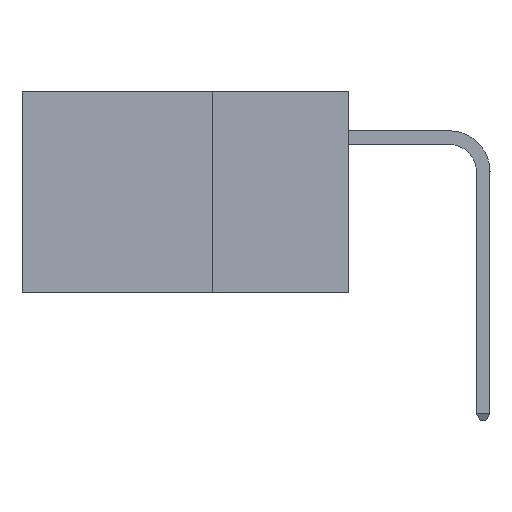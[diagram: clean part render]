
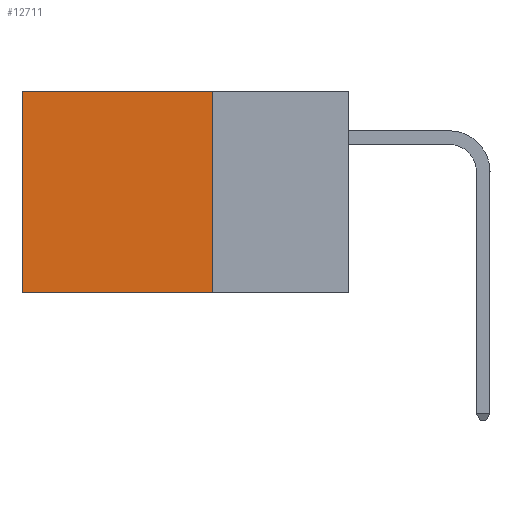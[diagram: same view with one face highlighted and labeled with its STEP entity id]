
A CAD part, left-side view. The second image highlights one B-rep face of the part: STEP entity #12711.
In plain terms, the highlighted planar face has unit normal (-1, 0, 0).
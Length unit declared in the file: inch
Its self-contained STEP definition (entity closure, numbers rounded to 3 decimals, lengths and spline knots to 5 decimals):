
#308 = EDGE_LOOP ( 'NONE', ( #20492, #718, #16041, #16776 ) ) ;
#398 = VERTEX_POINT ( 'NONE', #2685 ) ;
#718 = ORIENTED_EDGE ( 'NONE', *, *, #15885, .F. ) ;
#1490 = VECTOR ( 'NONE', #13937, 39.37008 ) ;
#2306 = CARTESIAN_POINT ( 'NONE',  ( 0.2875, 0.25, 0. ) ) ;
#2685 = CARTESIAN_POINT ( 'NONE',  ( 0.2875, 0.25, 0. ) ) ;
#4040 = DIRECTION ( 'NONE',  ( 0., 0., -1. ) ) ;
#4155 = EDGE_CURVE ( 'NONE', #398, #4259, #14075, .T. ) ;
#4259 = VERTEX_POINT ( 'NONE', #20538 ) ;
#4943 = VECTOR ( 'NONE', #10360, 39.37008 ) ;
#5597 = EDGE_CURVE ( 'NONE', #398, #18488, #15347, .T. ) ;
#5930 = AXIS2_PLACEMENT_3D ( 'NONE', #2306, #14076, #4040 ) ;
#7857 = DIRECTION ( 'NONE',  ( 0., 1., 0. ) ) ;
#8609 = EDGE_CURVE ( 'NONE', #4259, #18314, #19364, .T. ) ;
#8983 = CARTESIAN_POINT ( 'NONE',  ( 0.2875, 0.25, 0. ) ) ;
#10360 = DIRECTION ( 'NONE',  ( 0., 1., 0. ) ) ;
#12392 = PLANE ( 'NONE',  #5930 ) ;
#12711 = ADVANCED_FACE ( 'NONE', ( #15554 ), #12392, .F. ) ;
#13937 = DIRECTION ( 'NONE',  ( 0., 0., -1. ) ) ;
#14075 = LINE ( 'NONE', #15350, #4943 ) ;
#14076 = DIRECTION ( 'NONE',  ( 1., 0., 0. ) ) ;
#15347 = LINE ( 'NONE', #8983, #19241 ) ;
#15350 = CARTESIAN_POINT ( 'NONE',  ( 0.2875, 0.25, 0. ) ) ;
#15554 = FACE_OUTER_BOUND ( 'NONE', #308, .T. ) ;
#15842 = VECTOR ( 'NONE', #7857, 39.37008 ) ;
#15885 = EDGE_CURVE ( 'NONE', #18488, #18314, #20770, .T. ) ;
#16041 = ORIENTED_EDGE ( 'NONE', *, *, #5597, .F. ) ;
#16203 = CARTESIAN_POINT ( 'NONE',  ( 0.2875, 0.25, -0.37 ) ) ;
#16776 = ORIENTED_EDGE ( 'NONE', *, *, #4155, .T. ) ;
#17135 = CARTESIAN_POINT ( 'NONE',  ( 0.2875, 0.25, -0.37 ) ) ;
#17212 = CARTESIAN_POINT ( 'NONE',  ( 0.2875, 0.6, 0. ) ) ;
#18314 = VERTEX_POINT ( 'NONE', #18365 ) ;
#18365 = CARTESIAN_POINT ( 'NONE',  ( 0.2875, 0.6, -0.37 ) ) ;
#18488 = VERTEX_POINT ( 'NONE', #17135 ) ;
#19065 = DIRECTION ( 'NONE',  ( 0., 0., -1. ) ) ;
#19241 = VECTOR ( 'NONE', #19065, 39.37008 ) ;
#19364 = LINE ( 'NONE', #17212, #1490 ) ;
#20492 = ORIENTED_EDGE ( 'NONE', *, *, #8609, .T. ) ;
#20538 = CARTESIAN_POINT ( 'NONE',  ( 0.2875, 0.6, 0. ) ) ;
#20770 = LINE ( 'NONE', #16203, #15842 ) ;
